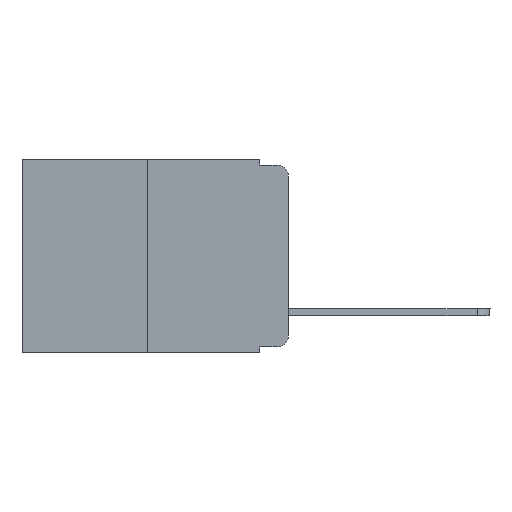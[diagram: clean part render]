
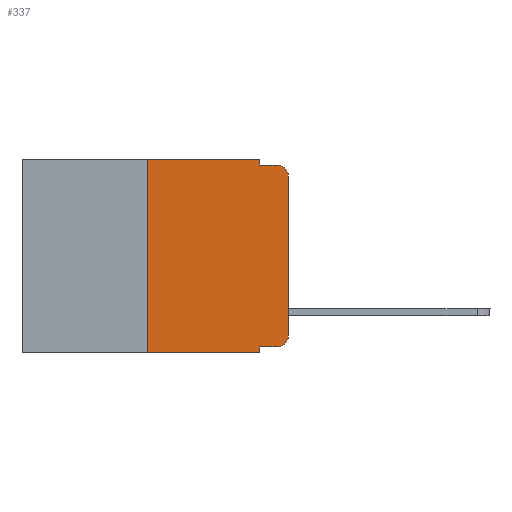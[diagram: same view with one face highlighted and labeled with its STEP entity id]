
A CAD part, left-side view. The second image highlights one B-rep face of the part: STEP entity #337.
In plain terms, the highlighted planar face has unit normal (-1, 0, 0).
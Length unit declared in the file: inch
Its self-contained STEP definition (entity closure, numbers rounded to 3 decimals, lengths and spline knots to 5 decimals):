
#142 = VECTOR ( 'NONE', #4463, 39.37008 ) ;
#337 = ADVANCED_FACE ( 'NONE', ( #719 ), #1916, .F. ) ;
#518 = LINE ( 'NONE', #8489, #142 ) ;
#719 = FACE_OUTER_BOUND ( 'NONE', #2050, .T. ) ;
#762 = VECTOR ( 'NONE', #2264, 39.37008 ) ;
#917 = DIRECTION ( 'NONE',  ( 1., 0., 0. ) ) ;
#1050 = EDGE_CURVE ( 'NONE', #6942, #5439, #6446, .T. ) ;
#1648 = CARTESIAN_POINT ( 'NONE',  ( 0., 0., -0.313 ) ) ;
#1707 = DIRECTION ( 'NONE',  ( 0., 0., 1. ) ) ;
#1813 = ORIENTED_EDGE ( 'NONE', *, *, #7223, .F. ) ;
#1916 = PLANE ( 'NONE',  #2179 ) ;
#2050 = EDGE_LOOP ( 'NONE', ( #4983, #9906, #10125, #3107, #8828, #1813, #10768, #6054, #5347, #10328 ) ) ;
#2153 = CIRCLE ( 'NONE', #5795, 0.02 ) ;
#2179 = AXIS2_PLACEMENT_3D ( 'NONE', #6950, #917, #13084 ) ;
#2264 = DIRECTION ( 'NONE',  ( 0., -1., 0. ) ) ;
#2364 = LINE ( 'NONE', #3568, #8115 ) ;
#2425 = VERTEX_POINT ( 'NONE', #9991 ) ;
#2526 = DIRECTION ( 'NONE',  ( 0., -1., 0. ) ) ;
#2614 = VECTOR ( 'NONE', #1707, 39.37008 ) ;
#2836 = VERTEX_POINT ( 'NONE', #7167 ) ;
#3098 = EDGE_CURVE ( 'NONE', #9914, #8230, #12294, .T. ) ;
#3107 = ORIENTED_EDGE ( 'NONE', *, *, #1050, .F. ) ;
#3187 = CARTESIAN_POINT ( 'NONE',  ( 0., 0.25, 0. ) ) ;
#3383 = CARTESIAN_POINT ( 'NONE',  ( 0., 0., -0.03 ) ) ;
#3394 = DIRECTION ( 'NONE',  ( -1., 0., 0. ) ) ;
#3466 = LINE ( 'NONE', #6432, #7661 ) ;
#3568 = CARTESIAN_POINT ( 'NONE',  ( 0., 0.051, -0.01 ) ) ;
#3801 = LINE ( 'NONE', #5814, #2614 ) ;
#4007 = CARTESIAN_POINT ( 'NONE',  ( 0., 0.051, -0.333 ) ) ;
#4463 = DIRECTION ( 'NONE',  ( 0., 0., -1. ) ) ;
#4665 = DIRECTION ( 'NONE',  ( 0., 0., -1. ) ) ;
#4670 = EDGE_CURVE ( 'NONE', #9381, #6942, #12515, .T. ) ;
#4953 = DIRECTION ( 'NONE',  ( 0., -1., 0. ) ) ;
#4983 = ORIENTED_EDGE ( 'NONE', *, *, #7237, .T. ) ;
#5274 = CARTESIAN_POINT ( 'NONE',  ( 0., 0.02, -0.01 ) ) ;
#5347 = ORIENTED_EDGE ( 'NONE', *, *, #5692, .T. ) ;
#5439 = VERTEX_POINT ( 'NONE', #5824 ) ;
#5692 = EDGE_CURVE ( 'NONE', #6882, #9914, #3466, .T. ) ;
#5779 = EDGE_CURVE ( 'NONE', #6882, #2836, #518, .T. ) ;
#5795 = AXIS2_PLACEMENT_3D ( 'NONE', #7375, #3394, #8425 ) ;
#5814 = CARTESIAN_POINT ( 'NONE',  ( 0., 0., 0. ) ) ;
#5824 = CARTESIAN_POINT ( 'NONE',  ( 0., 0.051, -0.01 ) ) ;
#6054 = ORIENTED_EDGE ( 'NONE', *, *, #5779, .F. ) ;
#6062 = VECTOR ( 'NONE', #12459, 39.37008 ) ;
#6376 = CARTESIAN_POINT ( 'NONE',  ( 0., 0.051, 0. ) ) ;
#6432 = CARTESIAN_POINT ( 'NONE',  ( 0., 0.051, -0.333 ) ) ;
#6446 = LINE ( 'NONE', #6376, #6062 ) ;
#6882 = VERTEX_POINT ( 'NONE', #4007 ) ;
#6942 = VERTEX_POINT ( 'NONE', #11442 ) ;
#6950 = CARTESIAN_POINT ( 'NONE',  ( 0., 0.473, 0. ) ) ;
#7167 = CARTESIAN_POINT ( 'NONE',  ( 0., 0.051, -0.343 ) ) ;
#7223 = EDGE_CURVE ( 'NONE', #2425, #9381, #11845, .T. ) ;
#7237 = EDGE_CURVE ( 'NONE', #8230, #9574, #3801, .T. ) ;
#7375 = CARTESIAN_POINT ( 'NONE',  ( 0., 0.02, -0.03 ) ) ;
#7661 = VECTOR ( 'NONE', #2526, 39.37008 ) ;
#7706 = DIRECTION ( 'NONE',  ( -1., 0., 0. ) ) ;
#7955 = CARTESIAN_POINT ( 'NONE',  ( 0., 0.25, 0. ) ) ;
#8054 = LINE ( 'NONE', #8988, #10935 ) ;
#8115 = VECTOR ( 'NONE', #12679, 39.37008 ) ;
#8133 = CARTESIAN_POINT ( 'NONE',  ( 0., 0.02, -0.333 ) ) ;
#8230 = VERTEX_POINT ( 'NONE', #1648 ) ;
#8425 = DIRECTION ( 'NONE',  ( 0., 0., -1. ) ) ;
#8489 = CARTESIAN_POINT ( 'NONE',  ( 0., 0.051, 0. ) ) ;
#8828 = ORIENTED_EDGE ( 'NONE', *, *, #4670, .F. ) ;
#8988 = CARTESIAN_POINT ( 'NONE',  ( 0., 0.473, -0.343 ) ) ;
#9381 = VERTEX_POINT ( 'NONE', #3187 ) ;
#9574 = VERTEX_POINT ( 'NONE', #3383 ) ;
#9698 = CARTESIAN_POINT ( 'NONE',  ( 0., 0.02, -0.313 ) ) ;
#9906 = ORIENTED_EDGE ( 'NONE', *, *, #12481, .T. ) ;
#9914 = VERTEX_POINT ( 'NONE', #8133 ) ;
#9991 = CARTESIAN_POINT ( 'NONE',  ( 0., 0.25, -0.343 ) ) ;
#10125 = ORIENTED_EDGE ( 'NONE', *, *, #12908, .F. ) ;
#10328 = ORIENTED_EDGE ( 'NONE', *, *, #3098, .T. ) ;
#10754 = VECTOR ( 'NONE', #10838, 39.37008 ) ;
#10768 = ORIENTED_EDGE ( 'NONE', *, *, #12703, .T. ) ;
#10838 = DIRECTION ( 'NONE',  ( 0., 0., 1. ) ) ;
#10935 = VECTOR ( 'NONE', #4953, 39.37008 ) ;
#11442 = CARTESIAN_POINT ( 'NONE',  ( 0., 0.051, 0. ) ) ;
#11845 = LINE ( 'NONE', #7955, #10754 ) ;
#12294 = CIRCLE ( 'NONE', #12503, 0.02 ) ;
#12384 = CARTESIAN_POINT ( 'NONE',  ( 0., 0.473, 0. ) ) ;
#12405 = VERTEX_POINT ( 'NONE', #5274 ) ;
#12459 = DIRECTION ( 'NONE',  ( 0., 0., -1. ) ) ;
#12481 = EDGE_CURVE ( 'NONE', #9574, #12405, #2153, .T. ) ;
#12503 = AXIS2_PLACEMENT_3D ( 'NONE', #9698, #7706, #4665 ) ;
#12515 = LINE ( 'NONE', #12384, #762 ) ;
#12679 = DIRECTION ( 'NONE',  ( 0., -1., 0. ) ) ;
#12703 = EDGE_CURVE ( 'NONE', #2425, #2836, #8054, .T. ) ;
#12908 = EDGE_CURVE ( 'NONE', #5439, #12405, #2364, .T. ) ;
#13084 = DIRECTION ( 'NONE',  ( 0., 0., -1. ) ) ;
